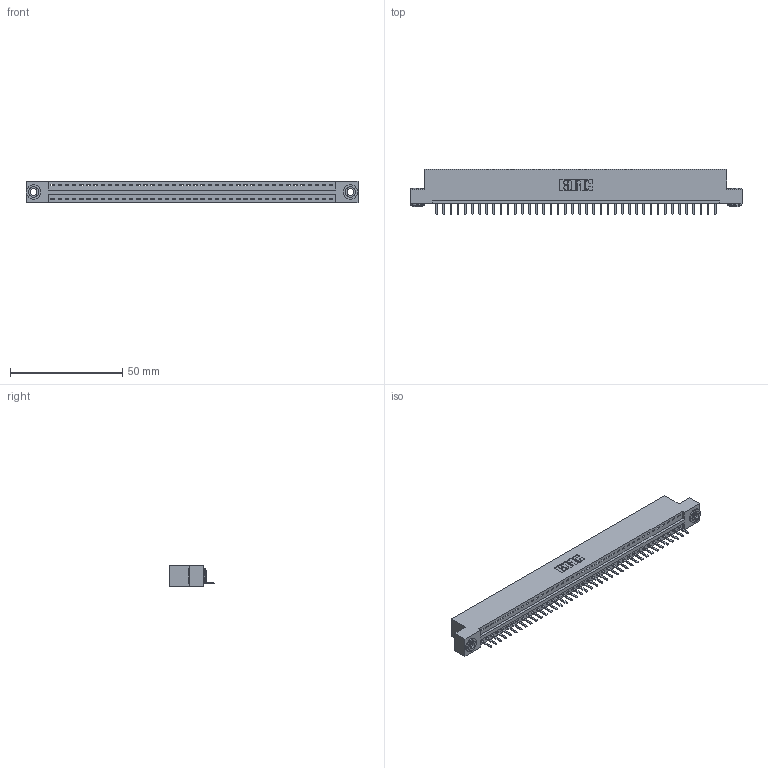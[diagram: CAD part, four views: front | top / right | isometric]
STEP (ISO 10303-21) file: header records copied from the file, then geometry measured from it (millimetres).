
FILE_DESCRIPTION (( 'STEP AP203' ), '1' );
FILE_NAME ('346-040-520-103.STEP', '2022-05-07T08:37:20', ( '' ), ( '' ), 'SwSTEP 2.0', 'SolidWorks 2020', '' );
FILE_SCHEMA (( 'CONFIG_CONTROL_DESIGN' ));
Length unit declared in the file: inch
Products named in the file (4): 345-250-002_345-250-002-102; 346-040-520-103; 345-292-001_345-293-120; 346 Part_Flush Mounting Lugs - 0.156 Dia-TH
Assembly tree (43 placements, depth 2):
  346-040-520-103
    346 Part_Flush Mounting Lugs - 0.156 Dia-TH
    345-292-001_345-293-120  x40
    345-250-002_345-250-002-102  x2
Bounding box: 147.57 x 20.02 x 9.4 mm (x, y, z)
Volume: 13998.6 mm3; surface area: 17342.2 mm2
Topology: 43 solids, 43 shells, 2654 faces, 7801 edges, 5090 vertices
Faces by surface type: plane 1780, cylinder 866, cone 8
Entity records: 26274 total; most frequent: CARTESIAN_POINT 4497, ORIENTED_EDGE 4450, DIRECTION 3987, EDGE_CURVE 2225, LINE 1905, VECTOR 1905, VERTEX_POINT 1478, AXIS2_PLACEMENT_3D 1041
